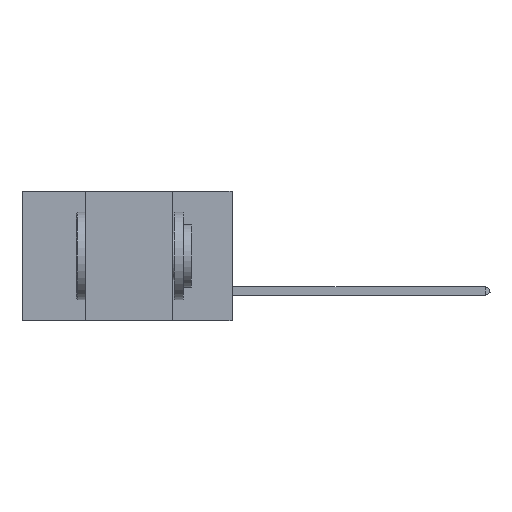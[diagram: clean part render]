
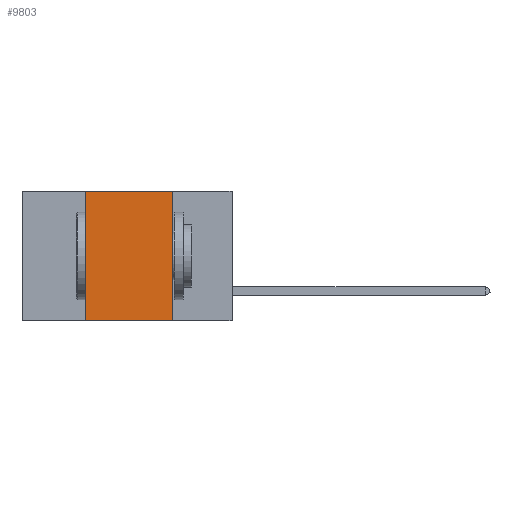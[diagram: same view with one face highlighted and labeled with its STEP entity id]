
A CAD part, left-side view. The second image highlights one B-rep face of the part: STEP entity #9803.
In plain terms, the highlighted planar face has unit normal (-1, 0, 0).
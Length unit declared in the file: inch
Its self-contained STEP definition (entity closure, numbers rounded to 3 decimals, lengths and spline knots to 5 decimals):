
#183 = CARTESIAN_POINT ( 'NONE',  ( 0., 0.17, 0. ) ) ;
#457 = VECTOR ( 'NONE', #3559, 39.37008 ) ;
#612 = LINE ( 'NONE', #9512, #3018 ) ;
#916 = CARTESIAN_POINT ( 'NONE',  ( 0., 0.17, 0. ) ) ;
#1319 = ORIENTED_EDGE ( 'NONE', *, *, #7321, .T. ) ;
#2329 = CARTESIAN_POINT ( 'NONE',  ( 0., 0.17, -0.37 ) ) ;
#2531 = CARTESIAN_POINT ( 'NONE',  ( 0., 0.42, 0. ) ) ;
#2592 = CARTESIAN_POINT ( 'NONE',  ( 0., 0.6, 0. ) ) ;
#2705 = LINE ( 'NONE', #2531, #457 ) ;
#2792 = VERTEX_POINT ( 'NONE', #10192 ) ;
#3018 = VECTOR ( 'NONE', #6675, 39.37008 ) ;
#3539 = DIRECTION ( 'NONE',  ( 1., 0., 0. ) ) ;
#3559 = DIRECTION ( 'NONE',  ( 0., 0., 1. ) ) ;
#3627 = DIRECTION ( 'NONE',  ( 0., -1., 0. ) ) ;
#3970 = VERTEX_POINT ( 'NONE', #2329 ) ;
#4916 = EDGE_CURVE ( 'NONE', #2792, #12662, #2705, .T. ) ;
#6554 = LINE ( 'NONE', #2592, #11989 ) ;
#6675 = DIRECTION ( 'NONE',  ( 0., -1., 0. ) ) ;
#6984 = EDGE_LOOP ( 'NONE', ( #9679, #11899, #9058, #1319 ) ) ;
#7107 = FACE_OUTER_BOUND ( 'NONE', #6984, .T. ) ;
#7176 = EDGE_CURVE ( 'NONE', #12662, #13070, #6554, .T. ) ;
#7207 = LINE ( 'NONE', #183, #7825 ) ;
#7321 = EDGE_CURVE ( 'NONE', #2792, #3970, #612, .T. ) ;
#7445 = CARTESIAN_POINT ( 'NONE',  ( 0., 0.42, 0. ) ) ;
#7486 = PLANE ( 'NONE',  #10647 ) ;
#7590 = CARTESIAN_POINT ( 'NONE',  ( 0., 0.6, 0. ) ) ;
#7825 = VECTOR ( 'NONE', #8333, 39.37008 ) ;
#8333 = DIRECTION ( 'NONE',  ( 0., 0., -1. ) ) ;
#9058 = ORIENTED_EDGE ( 'NONE', *, *, #4916, .F. ) ;
#9512 = CARTESIAN_POINT ( 'NONE',  ( 0., 0.6, -0.37 ) ) ;
#9679 = ORIENTED_EDGE ( 'NONE', *, *, #12058, .F. ) ;
#9803 = ADVANCED_FACE ( 'NONE', ( #7107 ), #7486, .F. ) ;
#10192 = CARTESIAN_POINT ( 'NONE',  ( 0., 0.42, -0.37 ) ) ;
#10647 = AXIS2_PLACEMENT_3D ( 'NONE', #7590, #3539, #11578 ) ;
#11578 = DIRECTION ( 'NONE',  ( 0., 0., -1. ) ) ;
#11899 = ORIENTED_EDGE ( 'NONE', *, *, #7176, .F. ) ;
#11989 = VECTOR ( 'NONE', #3627, 39.37008 ) ;
#12058 = EDGE_CURVE ( 'NONE', #13070, #3970, #7207, .T. ) ;
#12662 = VERTEX_POINT ( 'NONE', #7445 ) ;
#13070 = VERTEX_POINT ( 'NONE', #916 ) ;
